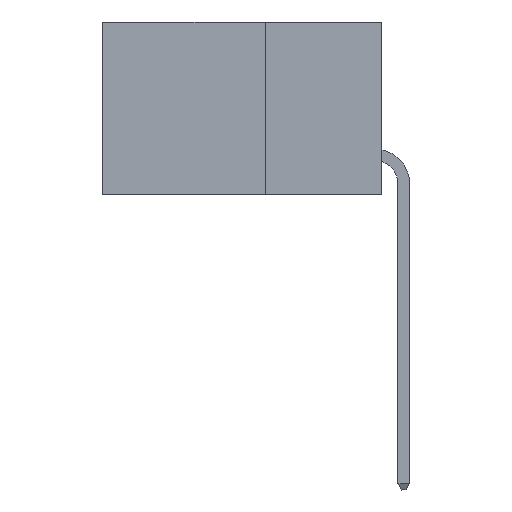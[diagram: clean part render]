
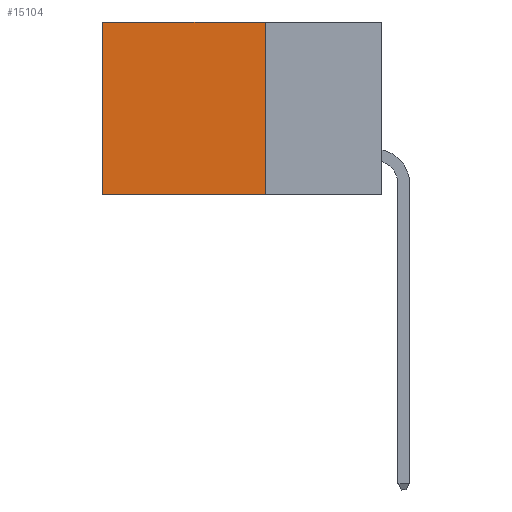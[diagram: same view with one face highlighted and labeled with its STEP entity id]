
A CAD part, left-side view. The second image highlights one B-rep face of the part: STEP entity #15104.
In plain terms, the highlighted planar face has unit normal (-1, 0, 0).
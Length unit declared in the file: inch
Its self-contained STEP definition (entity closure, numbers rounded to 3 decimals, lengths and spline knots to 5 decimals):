
#189 = VECTOR ( 'NONE', #5028, 39.37008 ) ;
#399 = AXIS2_PLACEMENT_3D ( 'NONE', #11009, #5991, #14671 ) ;
#613 = LINE ( 'NONE', #907, #16061 ) ;
#697 = EDGE_CURVE ( 'NONE', #2211, #14252, #613, .T. ) ;
#907 = CARTESIAN_POINT ( 'NONE',  ( 0.2875, 0.25, 0. ) ) ;
#1137 = DIRECTION ( 'NONE',  ( 0., 1., 0. ) ) ;
#1199 = FACE_OUTER_BOUND ( 'NONE', #14482, .T. ) ;
#2211 = VERTEX_POINT ( 'NONE', #10607 ) ;
#2221 = VERTEX_POINT ( 'NONE', #6869 ) ;
#2453 = ORIENTED_EDGE ( 'NONE', *, *, #697, .T. ) ;
#2720 = EDGE_CURVE ( 'NONE', #2211, #2221, #2965, .T. ) ;
#2895 = CARTESIAN_POINT ( 'NONE',  ( 0.2875, 0.6, 0. ) ) ;
#2965 = LINE ( 'NONE', #13938, #12159 ) ;
#3242 = ORIENTED_EDGE ( 'NONE', *, *, #12534, .F. ) ;
#3734 = CARTESIAN_POINT ( 'NONE',  ( 0.2875, 0.25, -0.37 ) ) ;
#3965 = LINE ( 'NONE', #4146, #13911 ) ;
#4146 = CARTESIAN_POINT ( 'NONE',  ( 0.2875, 0.6, 0. ) ) ;
#4933 = CARTESIAN_POINT ( 'NONE',  ( 0.2875, 0.6, -0.37 ) ) ;
#5028 = DIRECTION ( 'NONE',  ( 0., 1., 0. ) ) ;
#5991 = DIRECTION ( 'NONE',  ( 1., 0., 0. ) ) ;
#6869 = CARTESIAN_POINT ( 'NONE',  ( 0.2875, 0.25, -0.37 ) ) ;
#7793 = DIRECTION ( 'NONE',  ( 0., 0., -1. ) ) ;
#9159 = DIRECTION ( 'NONE',  ( 0., 0., -1. ) ) ;
#10607 = CARTESIAN_POINT ( 'NONE',  ( 0.2875, 0.25, 0. ) ) ;
#10749 = LINE ( 'NONE', #3734, #189 ) ;
#11009 = CARTESIAN_POINT ( 'NONE',  ( 0.2875, 0.25, 0. ) ) ;
#11858 = VERTEX_POINT ( 'NONE', #4933 ) ;
#12159 = VECTOR ( 'NONE', #7793, 39.37008 ) ;
#12424 = ORIENTED_EDGE ( 'NONE', *, *, #14185, .T. ) ;
#12534 = EDGE_CURVE ( 'NONE', #2221, #11858, #10749, .T. ) ;
#13427 = PLANE ( 'NONE',  #399 ) ;
#13911 = VECTOR ( 'NONE', #9159, 39.37008 ) ;
#13938 = CARTESIAN_POINT ( 'NONE',  ( 0.2875, 0.25, 0. ) ) ;
#14185 = EDGE_CURVE ( 'NONE', #14252, #11858, #3965, .T. ) ;
#14252 = VERTEX_POINT ( 'NONE', #2895 ) ;
#14482 = EDGE_LOOP ( 'NONE', ( #12424, #3242, #15236, #2453 ) ) ;
#14671 = DIRECTION ( 'NONE',  ( 0., 0., -1. ) ) ;
#15104 = ADVANCED_FACE ( 'NONE', ( #1199 ), #13427, .F. ) ;
#15236 = ORIENTED_EDGE ( 'NONE', *, *, #2720, .F. ) ;
#16061 = VECTOR ( 'NONE', #1137, 39.37008 ) ;
